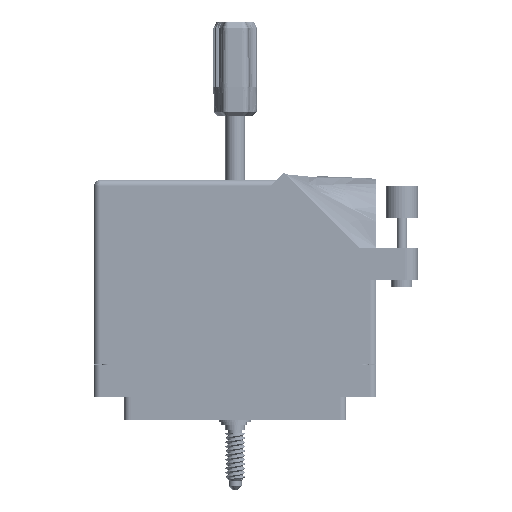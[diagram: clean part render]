
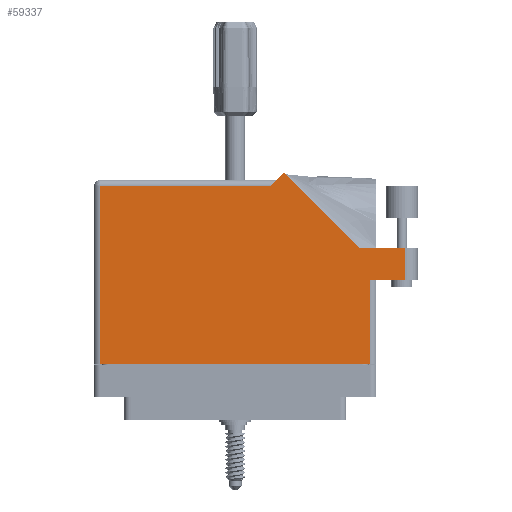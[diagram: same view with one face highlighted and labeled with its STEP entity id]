
A CAD part, front view. The second image highlights one B-rep face of the part: STEP entity #59337.
In plain terms, the highlighted face is planar.
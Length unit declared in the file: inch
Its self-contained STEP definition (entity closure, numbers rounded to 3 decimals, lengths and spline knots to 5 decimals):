
#506 = LINE ( 'NONE', #19638, #16297 ) ;
#589 = EDGE_CURVE ( 'NONE', #9043, #50786, #14697, .T. ) ;
#1348 = EDGE_CURVE ( 'NONE', #3457, #40589, #79454, .T. ) ;
#3457 = VERTEX_POINT ( 'NONE', #70917 ) ;
#6092 = ORIENTED_EDGE ( 'NONE', *, *, #1348, .T. ) ;
#6379 = VECTOR ( 'NONE', #14294, 39.37008 ) ;
#8906 = CARTESIAN_POINT ( 'NONE',  ( 0.399, 1.675, 0.617 ) ) ;
#9043 = VERTEX_POINT ( 'NONE', #13050 ) ;
#11420 = ORIENTED_EDGE ( 'NONE', *, *, #74870, .T. ) ;
#11758 = LINE ( 'NONE', #28084, #6379 ) ;
#12429 = VECTOR ( 'NONE', #20414, 39.37008 ) ;
#13050 = CARTESIAN_POINT ( 'NONE',  ( 1.297, 0.715, 0.617 ) ) ;
#13190 = CARTESIAN_POINT ( 'NONE',  ( 0.337, 1.613, 0.617 ) ) ;
#13641 = CARTESIAN_POINT ( 'NONE',  ( -1.359, 1.613, 0.617 ) ) ;
#13846 = CARTESIAN_POINT ( 'NONE',  ( 1.19342, 1.022, 0.617 ) ) ;
#14294 = DIRECTION ( 'NONE',  ( 0., 1., 0. ) ) ;
#14697 = LINE ( 'NONE', #59152, #60713 ) ;
#16297 = VECTOR ( 'NONE', #86343, 39.37008 ) ;
#16634 = ORIENTED_EDGE ( 'NONE', *, *, #56768, .T. ) ;
#17748 = VECTOR ( 'NONE', #43941, 39.37008 ) ;
#19427 = CARTESIAN_POINT ( 'NONE',  ( 0.46971, 1.74571, 0.617 ) ) ;
#19638 = CARTESIAN_POINT ( 'NONE',  ( -1.297, -0.1, 0.617 ) ) ;
#20414 = DIRECTION ( 'NONE',  ( 1., 0., 0. ) ) ;
#21314 = DIRECTION ( 'NONE',  ( 0., 0., -1. ) ) ;
#23713 = ORIENTED_EDGE ( 'NONE', *, *, #77988, .T. ) ;
#24040 = CARTESIAN_POINT ( 'NONE',  ( 1.634, 1.022, 0.617 ) ) ;
#26905 = CARTESIAN_POINT ( 'NONE',  ( -1.359, 1.675, 0.617 ) ) ;
#27138 = DIRECTION ( 'NONE',  ( -1., 0., 0. ) ) ;
#28084 = CARTESIAN_POINT ( 'NONE',  ( 1.634, 1.022, 0.617 ) ) ;
#30473 = AXIS2_PLACEMENT_3D ( 'NONE', #26905, #21314, #67527 ) ;
#31917 = LINE ( 'NONE', #8906, #65400 ) ;
#32095 = VECTOR ( 'NONE', #80794, 39.37008 ) ;
#34811 = CARTESIAN_POINT ( 'NONE',  ( 1.634, 0.715, 0.617 ) ) ;
#36587 = CARTESIAN_POINT ( 'NONE',  ( 1.759, 1.022, 0.617 ) ) ;
#36694 = VECTOR ( 'NONE', #50964, 39.37008 ) ;
#40260 = VERTEX_POINT ( 'NONE', #52395 ) ;
#40589 = VERTEX_POINT ( 'NONE', #75682 ) ;
#41473 = LINE ( 'NONE', #13846, #32095 ) ;
#43019 = LINE ( 'NONE', #64344, #36694 ) ;
#43941 = DIRECTION ( 'NONE',  ( -1., 0., 0. ) ) ;
#46967 = ORIENTED_EDGE ( 'NONE', *, *, #60335, .T. ) ;
#47888 = EDGE_LOOP ( 'NONE', ( #79873, #23713, #46967, #52892, #61427, #16634, #11420, #6092, #56553 ) ) ;
#50786 = VERTEX_POINT ( 'NONE', #34811 ) ;
#50964 = DIRECTION ( 'NONE',  ( 0., 1., 0. ) ) ;
#51273 = EDGE_CURVE ( 'NONE', #63074, #51351, #31917, .T. ) ;
#51351 = VERTEX_POINT ( 'NONE', #13190 ) ;
#52395 = CARTESIAN_POINT ( 'NONE',  ( -1.297, 1.613, 0.617 ) ) ;
#52892 = ORIENTED_EDGE ( 'NONE', *, *, #55836, .T. ) ;
#53173 = EDGE_CURVE ( 'NONE', #40589, #9043, #43019, .T. ) ;
#55808 = DIRECTION ( 'NONE',  ( -0.707, -0.707, 0. ) ) ;
#55836 = EDGE_CURVE ( 'NONE', #75177, #63074, #41473, .T. ) ;
#56444 = LINE ( 'NONE', #36587, #17748 ) ;
#56553 = ORIENTED_EDGE ( 'NONE', *, *, #53173, .T. ) ;
#56768 = EDGE_CURVE ( 'NONE', #51351, #40260, #66492, .T. ) ;
#59152 = CARTESIAN_POINT ( 'NONE',  ( 1.359, 0.715, 0.617 ) ) ;
#59337 = ADVANCED_FACE ( 'NONE', ( #59758 ), #60212, .F. ) ;
#59758 = FACE_OUTER_BOUND ( 'NONE', #47888, .T. ) ;
#60212 = PLANE ( 'NONE',  #30473 ) ;
#60335 = EDGE_CURVE ( 'NONE', #77849, #75177, #56444, .T. ) ;
#60713 = VECTOR ( 'NONE', #71511, 39.37008 ) ;
#61427 = ORIENTED_EDGE ( 'NONE', *, *, #51273, .T. ) ;
#61976 = CARTESIAN_POINT ( 'NONE',  ( 1.19342, 1.022, 0.617 ) ) ;
#63074 = VERTEX_POINT ( 'NONE', #19427 ) ;
#64344 = CARTESIAN_POINT ( 'NONE',  ( 1.297, 0.715, 0.617 ) ) ;
#65400 = VECTOR ( 'NONE', #55808, 39.37008 ) ;
#66492 = LINE ( 'NONE', #13641, #75878 ) ;
#66925 = CARTESIAN_POINT ( 'NONE',  ( -1.359, -0.1, 0.617 ) ) ;
#67527 = DIRECTION ( 'NONE',  ( -1., 0., 0. ) ) ;
#70917 = CARTESIAN_POINT ( 'NONE',  ( -1.297, -0.1, 0.617 ) ) ;
#71511 = DIRECTION ( 'NONE',  ( 1., 0., 0. ) ) ;
#74870 = EDGE_CURVE ( 'NONE', #40260, #3457, #506, .T. ) ;
#75177 = VERTEX_POINT ( 'NONE', #61976 ) ;
#75682 = CARTESIAN_POINT ( 'NONE',  ( 1.297, -0.1, 0.617 ) ) ;
#75878 = VECTOR ( 'NONE', #27138, 39.37008 ) ;
#77849 = VERTEX_POINT ( 'NONE', #24040 ) ;
#77988 = EDGE_CURVE ( 'NONE', #50786, #77849, #11758, .T. ) ;
#79454 = LINE ( 'NONE', #66925, #12429 ) ;
#79873 = ORIENTED_EDGE ( 'NONE', *, *, #589, .T. ) ;
#80794 = DIRECTION ( 'NONE',  ( -0.707, 0.707, 0. ) ) ;
#86343 = DIRECTION ( 'NONE',  ( 0., -1., 0. ) ) ;
